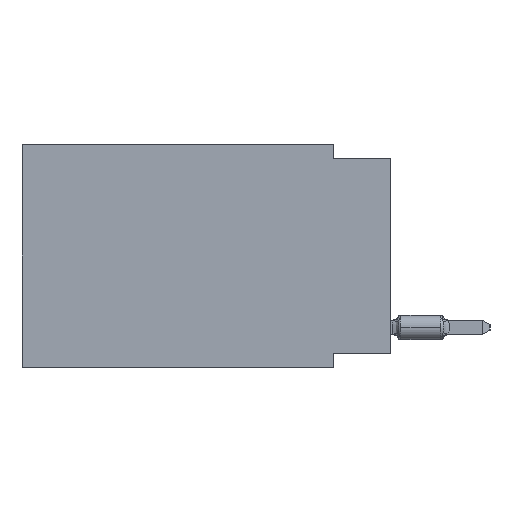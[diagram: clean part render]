
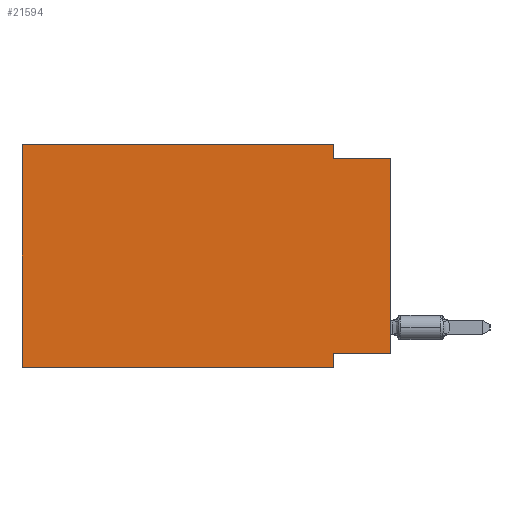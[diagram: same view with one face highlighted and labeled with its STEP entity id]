
A CAD part, left-side view. The second image highlights one B-rep face of the part: STEP entity #21594.
In plain terms, the highlighted planar face has unit normal (-1, 0, 0).
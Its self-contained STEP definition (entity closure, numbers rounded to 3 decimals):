
#385 = VECTOR ( 'NONE', #3159, 1000. ) ;
#443 = LINE ( 'NONE', #8374, #27908 ) ;
#663 = DIRECTION ( 'NONE',  ( 0., 0., -1. ) ) ;
#823 = EDGE_LOOP ( 'NONE', ( #22617, #16975, #11793, #15922, #26889, #13832, #1506, #19169 ) ) ;
#1506 = ORIENTED_EDGE ( 'NONE', *, *, #25678, .F. ) ;
#1682 = LINE ( 'NONE', #19947, #32777 ) ;
#2866 = CARTESIAN_POINT ( 'NONE',  ( 0., 2.54, -9.906 ) ) ;
#2943 = FACE_OUTER_BOUND ( 'NONE', #823, .T. ) ;
#3159 = DIRECTION ( 'NONE',  ( 0., -1., 0. ) ) ;
#3277 = LINE ( 'NONE', #14012, #30254 ) ;
#4055 = EDGE_CURVE ( 'NONE', #28777, #4527, #19469, .T. ) ;
#4215 = VECTOR ( 'NONE', #32801, 1000. ) ;
#4424 = VECTOR ( 'NONE', #29752, 1000. ) ;
#4527 = VERTEX_POINT ( 'NONE', #9842 ) ;
#5169 = VERTEX_POINT ( 'NONE', #25030 ) ;
#5460 = EDGE_CURVE ( 'NONE', #21505, #15350, #8175, .T. ) ;
#5642 = LINE ( 'NONE', #10896, #385 ) ;
#6283 = DIRECTION ( 'NONE',  ( 0., 0., 1. ) ) ;
#6588 = DIRECTION ( 'NONE',  ( 0., 0., 1. ) ) ;
#7382 = CARTESIAN_POINT ( 'NONE',  ( 0., 0., -0.635 ) ) ;
#8175 = LINE ( 'NONE', #16417, #4424 ) ;
#8226 = CARTESIAN_POINT ( 'NONE',  ( 0., 16.383, 0. ) ) ;
#8374 = CARTESIAN_POINT ( 'NONE',  ( 0., 0., -0.635 ) ) ;
#9792 = EDGE_CURVE ( 'NONE', #17379, #5169, #15074, .T. ) ;
#9842 = CARTESIAN_POINT ( 'NONE',  ( 0., 2.54, -9.271 ) ) ;
#10896 = CARTESIAN_POINT ( 'NONE',  ( 0., 16.383, 0. ) ) ;
#11793 = ORIENTED_EDGE ( 'NONE', *, *, #9792, .F. ) ;
#13832 = ORIENTED_EDGE ( 'NONE', *, *, #5460, .T. ) ;
#14012 = CARTESIAN_POINT ( 'NONE',  ( 0., 2.54, -9.906 ) ) ;
#14467 = VERTEX_POINT ( 'NONE', #7382 ) ;
#15074 = LINE ( 'NONE', #17524, #15421 ) ;
#15350 = VERTEX_POINT ( 'NONE', #2866 ) ;
#15421 = VECTOR ( 'NONE', #28061, 1000. ) ;
#15789 = EDGE_CURVE ( 'NONE', #25111, #17379, #5642, .T. ) ;
#15922 = ORIENTED_EDGE ( 'NONE', *, *, #15789, .F. ) ;
#16417 = CARTESIAN_POINT ( 'NONE',  ( 0., 16.383, -9.906 ) ) ;
#16426 = EDGE_CURVE ( 'NONE', #5169, #14467, #443, .T. ) ;
#16975 = ORIENTED_EDGE ( 'NONE', *, *, #16426, .F. ) ;
#17379 = VERTEX_POINT ( 'NONE', #19493 ) ;
#17524 = CARTESIAN_POINT ( 'NONE',  ( 0., 2.54, 0. ) ) ;
#18041 = VECTOR ( 'NONE', #6588, 1000. ) ;
#19169 = ORIENTED_EDGE ( 'NONE', *, *, #4055, .F. ) ;
#19242 = DIRECTION ( 'NONE',  ( 0., -1., 0. ) ) ;
#19469 = LINE ( 'NONE', #22106, #4215 ) ;
#19493 = CARTESIAN_POINT ( 'NONE',  ( 0., 2.54, 0. ) ) ;
#19668 = AXIS2_PLACEMENT_3D ( 'NONE', #8226, #26652, #27159 ) ;
#19947 = CARTESIAN_POINT ( 'NONE',  ( 0., 0., 0. ) ) ;
#20084 = CARTESIAN_POINT ( 'NONE',  ( 0., 16.383, 0. ) ) ;
#21505 = VERTEX_POINT ( 'NONE', #22515 ) ;
#21594 = ADVANCED_FACE ( 'NONE', ( #2943 ), #31912, .F. ) ;
#22106 = CARTESIAN_POINT ( 'NONE',  ( 0., 0., -9.271 ) ) ;
#22515 = CARTESIAN_POINT ( 'NONE',  ( 0., 16.383, -9.906 ) ) ;
#22617 = ORIENTED_EDGE ( 'NONE', *, *, #34116, .T. ) ;
#23346 = EDGE_CURVE ( 'NONE', #21505, #25111, #30102, .T. ) ;
#25030 = CARTESIAN_POINT ( 'NONE',  ( 0., 2.54, -0.635 ) ) ;
#25111 = VERTEX_POINT ( 'NONE', #31776 ) ;
#25678 = EDGE_CURVE ( 'NONE', #4527, #15350, #3277, .T. ) ;
#25903 = CARTESIAN_POINT ( 'NONE',  ( 0., 0., -9.271 ) ) ;
#26652 = DIRECTION ( 'NONE',  ( 1., 0., 0. ) ) ;
#26889 = ORIENTED_EDGE ( 'NONE', *, *, #23346, .F. ) ;
#27159 = DIRECTION ( 'NONE',  ( 0., 0., -1. ) ) ;
#27908 = VECTOR ( 'NONE', #19242, 1000. ) ;
#28061 = DIRECTION ( 'NONE',  ( 0., 0., -1. ) ) ;
#28777 = VERTEX_POINT ( 'NONE', #25903 ) ;
#29752 = DIRECTION ( 'NONE',  ( 0., -1., 0. ) ) ;
#30102 = LINE ( 'NONE', #20084, #18041 ) ;
#30254 = VECTOR ( 'NONE', #663, 1000. ) ;
#31776 = CARTESIAN_POINT ( 'NONE',  ( 0., 16.383, 0. ) ) ;
#31912 = PLANE ( 'NONE',  #19668 ) ;
#32777 = VECTOR ( 'NONE', #6283, 1000. ) ;
#32801 = DIRECTION ( 'NONE',  ( 0., 1., 0. ) ) ;
#34116 = EDGE_CURVE ( 'NONE', #28777, #14467, #1682, .T. ) ;
